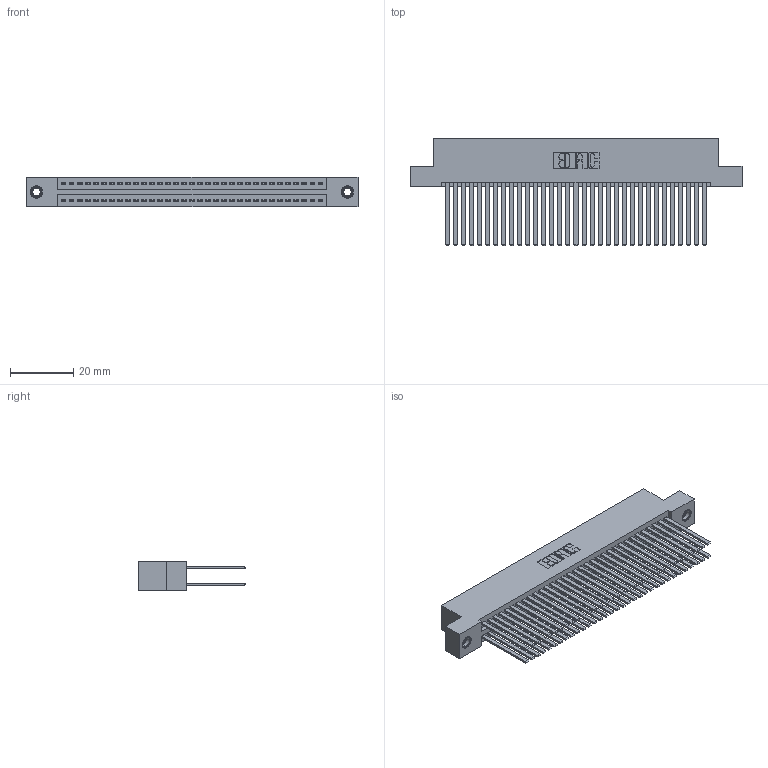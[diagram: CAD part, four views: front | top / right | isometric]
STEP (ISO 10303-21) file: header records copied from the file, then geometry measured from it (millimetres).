
FILE_DESCRIPTION (( 'STEP AP203' ), '1' );
FILE_NAME ('345-066-544-207.STEP', '2019-10-30T17:38:32', ( '' ), ( '' ), 'SwSTEP 2.0', 'SolidWorks 2016', '' );
FILE_SCHEMA (( 'CONFIG_CONTROL_DESIGN' ));
Length unit declared in the file: inch
Products named in the file (4): 345-250-001_345-250-005-103; 345 Part_Flush Mounting Lugs - 0.156 Dia-TI; 345-066-544-207; 345-292-001_345-293-144
Assembly tree (69 placements, depth 2):
  345-066-544-207
    345 Part_Flush Mounting Lugs - 0.156 Dia-TI
    345-292-001_345-293-144  x66
    345-250-001_345-250-005-103  x2
Bounding box: 105.03 x 33.96 x 9.4 mm (x, y, z)
Volume: 11030.8 mm3; surface area: 18870.6 mm2
Topology: 69 solids, 69 shells, 3090 faces, 9123 edges, 5986 vertices
Faces by surface type: plane 2026, cylinder 1048, cone 12, torus 4
Entity records: 28106 total; most frequent: CARTESIAN_POINT 4699, ORIENTED_EDGE 4626, DIRECTION 4179, EDGE_CURVE 2313, VECTOR 2033, LINE 2033, VERTEX_POINT 1536, AXIS2_PLACEMENT_3D 1073
